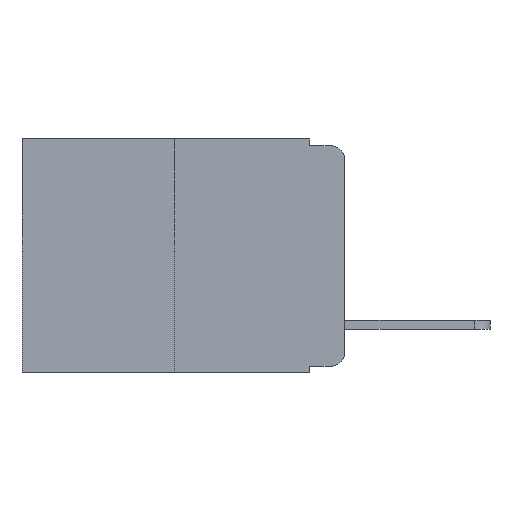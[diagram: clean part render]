
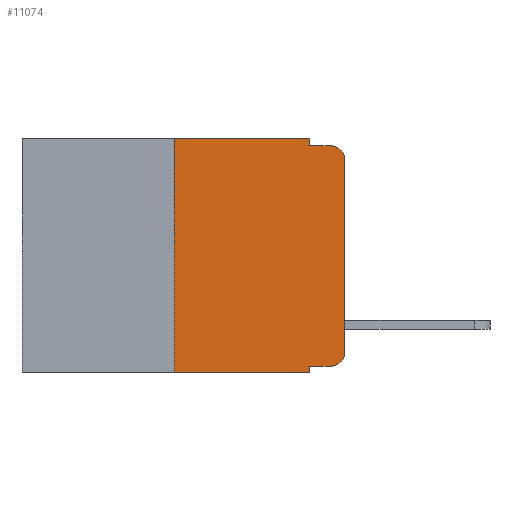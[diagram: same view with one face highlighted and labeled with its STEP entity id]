
A CAD part, left-side view. The second image highlights one B-rep face of the part: STEP entity #11074.
In plain terms, the highlighted planar face has unit normal (-1, 0, 0).
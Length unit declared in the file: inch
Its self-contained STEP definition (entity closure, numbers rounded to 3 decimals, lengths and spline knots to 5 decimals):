
#379 = DIRECTION ( 'NONE',  ( 0., 0., -1. ) ) ;
#539 = VERTEX_POINT ( 'NONE', #6691 ) ;
#1477 = DIRECTION ( 'NONE',  ( 0., -1., 0. ) ) ;
#2979 = ORIENTED_EDGE ( 'NONE', *, *, #9198, .T. ) ;
#3089 = PLANE ( 'NONE',  #15450 ) ;
#3701 = EDGE_CURVE ( 'NONE', #11388, #4149, #13288, .T. ) ;
#4048 = CIRCLE ( 'NONE', #18789, 0.02 ) ;
#4059 = ORIENTED_EDGE ( 'NONE', *, *, #13674, .F. ) ;
#4146 = VERTEX_POINT ( 'NONE', #18592 ) ;
#4149 = VERTEX_POINT ( 'NONE', #16782 ) ;
#4226 = CARTESIAN_POINT ( 'NONE',  ( 0., 0., -0.03 ) ) ;
#4645 = VECTOR ( 'NONE', #18450, 39.37008 ) ;
#4806 = DIRECTION ( 'NONE',  ( 0., 0., -1. ) ) ;
#5044 = LINE ( 'NONE', #15317, #8833 ) ;
#5570 = CARTESIAN_POINT ( 'NONE',  ( 0., 0.051, 0. ) ) ;
#5574 = DIRECTION ( 'NONE',  ( 0., 0., 1. ) ) ;
#6376 = LINE ( 'NONE', #20509, #10637 ) ;
#6598 = VERTEX_POINT ( 'NONE', #4226 ) ;
#6674 = EDGE_CURVE ( 'NONE', #14523, #539, #6376, .T. ) ;
#6684 = CARTESIAN_POINT ( 'NONE',  ( 0., 0.051, -0.333 ) ) ;
#6691 = CARTESIAN_POINT ( 'NONE',  ( 0., 0.051, -0.343 ) ) ;
#7073 = EDGE_CURVE ( 'NONE', #14043, #14369, #5044, .T. ) ;
#7421 = ORIENTED_EDGE ( 'NONE', *, *, #8134, .F. ) ;
#7425 = CARTESIAN_POINT ( 'NONE',  ( 0., 0., 0. ) ) ;
#7786 = LINE ( 'NONE', #8167, #15156 ) ;
#7910 = ORIENTED_EDGE ( 'NONE', *, *, #7073, .F. ) ;
#7930 = CIRCLE ( 'NONE', #14417, 0.02 ) ;
#8134 = EDGE_CURVE ( 'NONE', #14369, #13287, #10249, .T. ) ;
#8167 = CARTESIAN_POINT ( 'NONE',  ( 0., 0.473, 0. ) ) ;
#8410 = VECTOR ( 'NONE', #10668, 39.37008 ) ;
#8428 = ORIENTED_EDGE ( 'NONE', *, *, #3701, .F. ) ;
#8833 = VECTOR ( 'NONE', #15560, 39.37008 ) ;
#8856 = DIRECTION ( 'NONE',  ( 0., 0., -1. ) ) ;
#8905 = DIRECTION ( 'NONE',  ( -1., 0., 0. ) ) ;
#8916 = ORIENTED_EDGE ( 'NONE', *, *, #15902, .T. ) ;
#8924 = CARTESIAN_POINT ( 'NONE',  ( 0., 0.02, -0.03 ) ) ;
#8961 = LINE ( 'NONE', #16985, #4645 ) ;
#9198 = EDGE_CURVE ( 'NONE', #6598, #13287, #7930, .T. ) ;
#9357 = DIRECTION ( 'NONE',  ( -1., 0., 0. ) ) ;
#9438 = ORIENTED_EDGE ( 'NONE', *, *, #6674, .F. ) ;
#9876 = EDGE_CURVE ( 'NONE', #14523, #4146, #18758, .T. ) ;
#10249 = LINE ( 'NONE', #18404, #13916 ) ;
#10293 = EDGE_CURVE ( 'NONE', #14756, #6598, #16705, .T. ) ;
#10451 = ORIENTED_EDGE ( 'NONE', *, *, #9876, .T. ) ;
#10637 = VECTOR ( 'NONE', #379, 39.37008 ) ;
#10668 = DIRECTION ( 'NONE',  ( 0., 0., 1. ) ) ;
#10699 = ORIENTED_EDGE ( 'NONE', *, *, #10293, .T. ) ;
#10705 = VECTOR ( 'NONE', #16076, 39.37008 ) ;
#10975 = ORIENTED_EDGE ( 'NONE', *, *, #10990, .T. ) ;
#10990 = EDGE_CURVE ( 'NONE', #4146, #14756, #4048, .T. ) ;
#11074 = ADVANCED_FACE ( 'NONE', ( #14803 ), #3089, .F. ) ;
#11388 = VERTEX_POINT ( 'NONE', #18213 ) ;
#13287 = VERTEX_POINT ( 'NONE', #15233 ) ;
#13288 = LINE ( 'NONE', #19505, #20549 ) ;
#13674 = EDGE_CURVE ( 'NONE', #4149, #14043, #7786, .T. ) ;
#13916 = VECTOR ( 'NONE', #16671, 39.37008 ) ;
#14043 = VERTEX_POINT ( 'NONE', #5570 ) ;
#14280 = CARTESIAN_POINT ( 'NONE',  ( 0., 0.051, -0.333 ) ) ;
#14367 = DIRECTION ( 'NONE',  ( 1., 0., 0. ) ) ;
#14369 = VERTEX_POINT ( 'NONE', #15544 ) ;
#14417 = AXIS2_PLACEMENT_3D ( 'NONE', #8924, #8905, #8856 ) ;
#14523 = VERTEX_POINT ( 'NONE', #14280 ) ;
#14756 = VERTEX_POINT ( 'NONE', #19059 ) ;
#14803 = FACE_OUTER_BOUND ( 'NONE', #17869, .T. ) ;
#15156 = VECTOR ( 'NONE', #1477, 39.37008 ) ;
#15233 = CARTESIAN_POINT ( 'NONE',  ( 0., 0.02, -0.01 ) ) ;
#15317 = CARTESIAN_POINT ( 'NONE',  ( 0., 0.051, 0. ) ) ;
#15450 = AXIS2_PLACEMENT_3D ( 'NONE', #18776, #14367, #4806 ) ;
#15544 = CARTESIAN_POINT ( 'NONE',  ( 0., 0.051, -0.01 ) ) ;
#15560 = DIRECTION ( 'NONE',  ( 0., 0., -1. ) ) ;
#15902 = EDGE_CURVE ( 'NONE', #11388, #539, #8961, .T. ) ;
#16076 = DIRECTION ( 'NONE',  ( 0., -1., 0. ) ) ;
#16671 = DIRECTION ( 'NONE',  ( 0., -1., 0. ) ) ;
#16705 = LINE ( 'NONE', #7425, #8410 ) ;
#16782 = CARTESIAN_POINT ( 'NONE',  ( 0., 0.25, 0. ) ) ;
#16985 = CARTESIAN_POINT ( 'NONE',  ( 0., 0.473, -0.343 ) ) ;
#17869 = EDGE_LOOP ( 'NONE', ( #10699, #2979, #7421, #7910, #4059, #8428, #8916, #9438, #10451, #10975 ) ) ;
#18213 = CARTESIAN_POINT ( 'NONE',  ( 0., 0.25, -0.343 ) ) ;
#18404 = CARTESIAN_POINT ( 'NONE',  ( 0., 0.051, -0.01 ) ) ;
#18450 = DIRECTION ( 'NONE',  ( 0., -1., 0. ) ) ;
#18550 = CARTESIAN_POINT ( 'NONE',  ( 0., 0.02, -0.313 ) ) ;
#18592 = CARTESIAN_POINT ( 'NONE',  ( 0., 0.02, -0.333 ) ) ;
#18758 = LINE ( 'NONE', #6684, #10705 ) ;
#18776 = CARTESIAN_POINT ( 'NONE',  ( 0., 0.473, 0. ) ) ;
#18789 = AXIS2_PLACEMENT_3D ( 'NONE', #18550, #9357, #19915 ) ;
#19059 = CARTESIAN_POINT ( 'NONE',  ( 0., 0., -0.313 ) ) ;
#19505 = CARTESIAN_POINT ( 'NONE',  ( 0., 0.25, 0. ) ) ;
#19915 = DIRECTION ( 'NONE',  ( 0., 0., -1. ) ) ;
#20509 = CARTESIAN_POINT ( 'NONE',  ( 0., 0.051, 0. ) ) ;
#20549 = VECTOR ( 'NONE', #5574, 39.37008 ) ;
